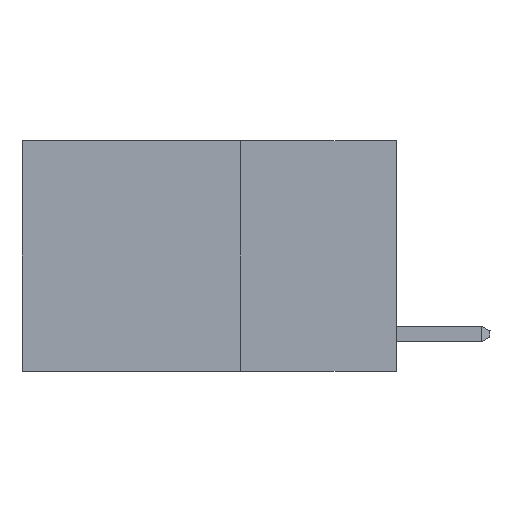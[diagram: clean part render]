
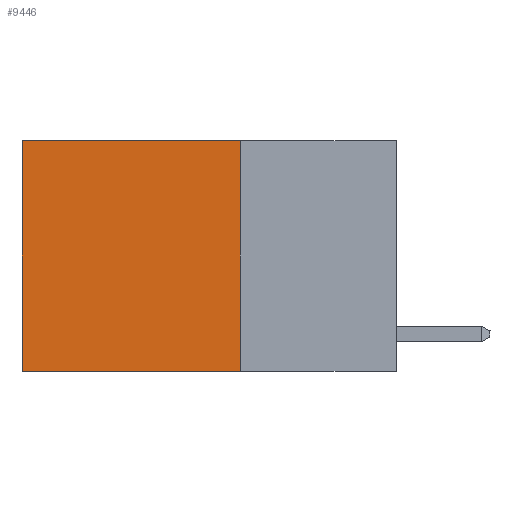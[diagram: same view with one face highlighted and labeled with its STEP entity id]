
A CAD part, left-side view. The second image highlights one B-rep face of the part: STEP entity #9446.
In plain terms, the highlighted planar face has unit normal (-1, 0, 0).
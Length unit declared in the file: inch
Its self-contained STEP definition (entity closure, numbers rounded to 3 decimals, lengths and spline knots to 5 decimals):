
#412 = ORIENTED_EDGE ( 'NONE', *, *, #2937, .F. ) ;
#542 = DIRECTION ( 'NONE',  ( 1., 0., 0. ) ) ;
#1423 = VERTEX_POINT ( 'NONE', #11778 ) ;
#1450 = VECTOR ( 'NONE', #9188, 39.37008 ) ;
#1998 = DIRECTION ( 'NONE',  ( 0., 1., 0. ) ) ;
#2627 = EDGE_LOOP ( 'NONE', ( #7995, #412, #14488, #18065 ) ) ;
#2937 = EDGE_CURVE ( 'NONE', #5629, #1423, #16681, .T. ) ;
#3256 = LINE ( 'NONE', #13810, #1450 ) ;
#3283 = CARTESIAN_POINT ( 'NONE',  ( 0.2625, 0.25, -0.37 ) ) ;
#3419 = FACE_OUTER_BOUND ( 'NONE', #2627, .T. ) ;
#3480 = DIRECTION ( 'NONE',  ( 0., 0., -1. ) ) ;
#3699 = CARTESIAN_POINT ( 'NONE',  ( 0.2625, 0.25, 0. ) ) ;
#5629 = VERTEX_POINT ( 'NONE', #3283 ) ;
#6294 = CARTESIAN_POINT ( 'NONE',  ( 0.2625, 0.6, 0. ) ) ;
#6661 = VECTOR ( 'NONE', #19022, 39.37008 ) ;
#6913 = LINE ( 'NONE', #17361, #6661 ) ;
#7020 = CARTESIAN_POINT ( 'NONE',  ( 0.2625, 0.6, 0. ) ) ;
#7995 = ORIENTED_EDGE ( 'NONE', *, *, #17358, .T. ) ;
#9188 = DIRECTION ( 'NONE',  ( 0., 1., 0. ) ) ;
#9446 = ADVANCED_FACE ( 'NONE', ( #3419 ), #17943, .F. ) ;
#9586 = VERTEX_POINT ( 'NONE', #3699 ) ;
#9749 = VERTEX_POINT ( 'NONE', #7020 ) ;
#10022 = AXIS2_PLACEMENT_3D ( 'NONE', #13495, #542, #12146 ) ;
#11778 = CARTESIAN_POINT ( 'NONE',  ( 0.2625, 0.6, -0.37 ) ) ;
#12146 = DIRECTION ( 'NONE',  ( 0., 0., -1. ) ) ;
#12695 = EDGE_CURVE ( 'NONE', #9586, #5629, #6913, .T. ) ;
#12958 = VECTOR ( 'NONE', #1998, 39.37008 ) ;
#13495 = CARTESIAN_POINT ( 'NONE',  ( 0.2625, 0.25, 0. ) ) ;
#13543 = VECTOR ( 'NONE', #3480, 39.37008 ) ;
#13810 = CARTESIAN_POINT ( 'NONE',  ( 0.2625, 0.25, 0. ) ) ;
#14488 = ORIENTED_EDGE ( 'NONE', *, *, #12695, .F. ) ;
#16659 = LINE ( 'NONE', #6294, #13543 ) ;
#16681 = LINE ( 'NONE', #16857, #12958 ) ;
#16857 = CARTESIAN_POINT ( 'NONE',  ( 0.2625, 0.25, -0.37 ) ) ;
#17358 = EDGE_CURVE ( 'NONE', #9749, #1423, #16659, .T. ) ;
#17361 = CARTESIAN_POINT ( 'NONE',  ( 0.2625, 0.25, 0. ) ) ;
#17843 = EDGE_CURVE ( 'NONE', #9586, #9749, #3256, .T. ) ;
#17943 = PLANE ( 'NONE',  #10022 ) ;
#18065 = ORIENTED_EDGE ( 'NONE', *, *, #17843, .T. ) ;
#19022 = DIRECTION ( 'NONE',  ( 0., 0., -1. ) ) ;
